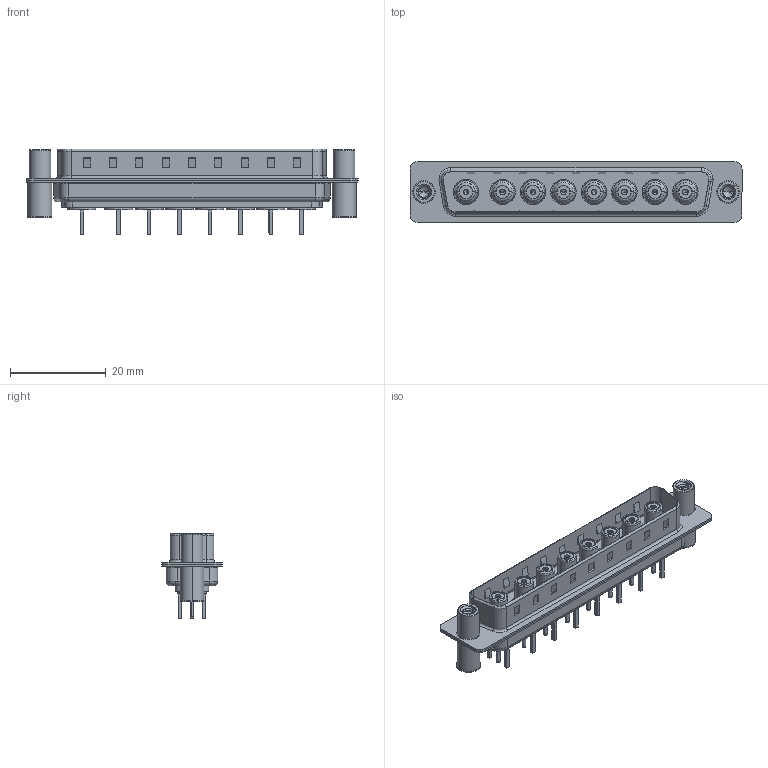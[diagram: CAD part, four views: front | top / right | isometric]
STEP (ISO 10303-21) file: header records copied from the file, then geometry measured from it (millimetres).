
FILE_DESCRIPTION (( 'STEP AP203' ), '1' );
FILE_NAME ('627-8W8-624-7T4.STEP', '2019-05-28T06:15:57', ( '' ), ( '' ), 'SwSTEP 2.0', 'SolidWorks 2016', '' );
FILE_SCHEMA (( 'CONFIG_CONTROL_DESIGN' ));
Length unit declared in the file: millimetre
Products named in the file (11): Insulator Socket; Locking Collar; 627-8W8-624-7T4; 627Combo Threaded Standoff and Board Spacer_4; Co-Ax Jack Assy_S; Insulator Socket 2; 627Combo Shell Front_37 Contacts; Socket_Str; 627Combo Housing_8W8; 627Combo Shell Rear_37 Contacts; Co-Ax Jack_Straight PC Tail
Assembly tree (18 placements, depth 3):
  627-8W8-624-7T4
    627Combo Housing_8W8
    627Combo Shell Rear_37 Contacts
    627Combo Shell Front_37 Contacts
    627Combo Threaded Standoff and Board Spacer_4  x2
    Co-Ax Jack Assy_S  x8
      Co-Ax Jack_Straight PC Tail
      Insulator Socket
      Insulator Socket 2
      Locking Collar
      Socket_Str
Bounding box: 69.3 x 12.6 x 17.9 mm (x, y, z)
Volume: 4239.2 mm3; surface area: 12996.6 mm2
Topology: 45 solids, 45 shells, 1386 faces, 3275 edges, 2052 vertices
Faces by surface type: plane 585, cylinder 569, cone 102, torus 86, bspline 28, sphere 16
Entity records: 20467 total; most frequent: CARTESIAN_POINT 5295, DIRECTION 2955, ORIENTED_EDGE 2824, EDGE_CURVE 1412, AXIS2_PLACEMENT_3D 1073, VERTEX_POINT 895, VECTOR 809, LINE 809
